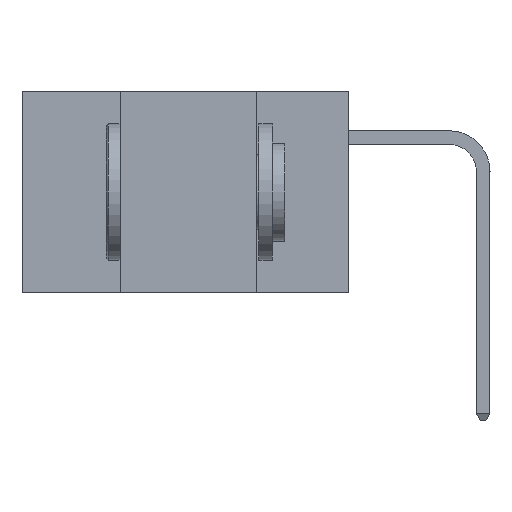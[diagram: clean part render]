
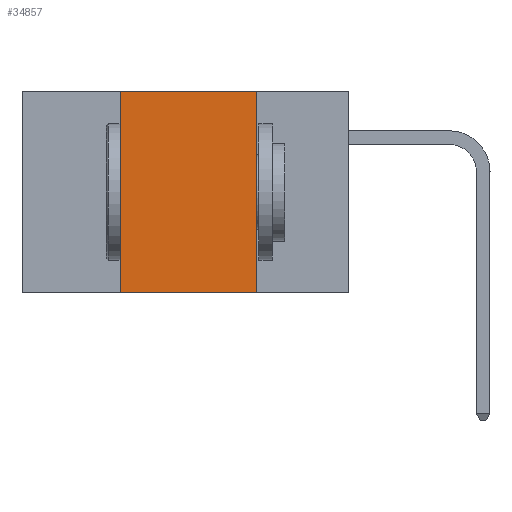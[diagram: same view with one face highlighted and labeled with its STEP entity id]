
A CAD part, left-side view. The second image highlights one B-rep face of the part: STEP entity #34857.
In plain terms, the highlighted planar face has unit normal (-1, 0, 0).
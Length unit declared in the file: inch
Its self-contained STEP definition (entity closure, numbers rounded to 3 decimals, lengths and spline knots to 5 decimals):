
#494 = LINE ( 'NONE', #39666, #38726 ) ;
#1566 = CARTESIAN_POINT ( 'NONE',  ( 0., 0.42, -0.37 ) ) ;
#3999 = VECTOR ( 'NONE', #14563, 39.37008 ) ;
#4906 = EDGE_CURVE ( 'NONE', #32123, #40632, #26420, .T. ) ;
#5770 = LINE ( 'NONE', #21380, #45044 ) ;
#10221 = AXIS2_PLACEMENT_3D ( 'NONE', #17290, #43224, #21131 ) ;
#13733 = PLANE ( 'NONE',  #10221 ) ;
#14563 = DIRECTION ( 'NONE',  ( 0., -1., 0. ) ) ;
#15925 = ORIENTED_EDGE ( 'NONE', *, *, #32417, .F. ) ;
#17290 = CARTESIAN_POINT ( 'NONE',  ( 0., 0.6, 0. ) ) ;
#19367 = EDGE_LOOP ( 'NONE', ( #20616, #15925, #19670, #27482 ) ) ;
#19670 = ORIENTED_EDGE ( 'NONE', *, *, #33658, .F. ) ;
#20616 = ORIENTED_EDGE ( 'NONE', *, *, #44656, .F. ) ;
#21131 = DIRECTION ( 'NONE',  ( 0., 0., -1. ) ) ;
#21380 = CARTESIAN_POINT ( 'NONE',  ( 0., 0.42, 0. ) ) ;
#22202 = CARTESIAN_POINT ( 'NONE',  ( 0., 0.42, 0. ) ) ;
#25004 = DIRECTION ( 'NONE',  ( 0., 0., -1. ) ) ;
#26420 = LINE ( 'NONE', #29782, #35036 ) ;
#27482 = ORIENTED_EDGE ( 'NONE', *, *, #4906, .T. ) ;
#28075 = CARTESIAN_POINT ( 'NONE',  ( 0., 0.17, -0.37 ) ) ;
#28185 = CARTESIAN_POINT ( 'NONE',  ( 0., 0.17, 0. ) ) ;
#29782 = CARTESIAN_POINT ( 'NONE',  ( 0., 0.6, -0.37 ) ) ;
#32123 = VERTEX_POINT ( 'NONE', #1566 ) ;
#32417 = EDGE_CURVE ( 'NONE', #36283, #41343, #42188, .T. ) ;
#33658 = EDGE_CURVE ( 'NONE', #32123, #36283, #5770, .T. ) ;
#34857 = ADVANCED_FACE ( 'NONE', ( #38551 ), #13733, .F. ) ;
#35036 = VECTOR ( 'NONE', #40934, 39.37008 ) ;
#36283 = VERTEX_POINT ( 'NONE', #22202 ) ;
#36633 = CARTESIAN_POINT ( 'NONE',  ( 0., 0.6, 0. ) ) ;
#38551 = FACE_OUTER_BOUND ( 'NONE', #19367, .T. ) ;
#38726 = VECTOR ( 'NONE', #25004, 39.37008 ) ;
#39666 = CARTESIAN_POINT ( 'NONE',  ( 0., 0.17, 0. ) ) ;
#40632 = VERTEX_POINT ( 'NONE', #28075 ) ;
#40934 = DIRECTION ( 'NONE',  ( 0., -1., 0. ) ) ;
#41343 = VERTEX_POINT ( 'NONE', #28185 ) ;
#42188 = LINE ( 'NONE', #36633, #3999 ) ;
#43224 = DIRECTION ( 'NONE',  ( 1., 0., 0. ) ) ;
#44656 = EDGE_CURVE ( 'NONE', #41343, #40632, #494, .T. ) ;
#45044 = VECTOR ( 'NONE', #47178, 39.37008 ) ;
#47178 = DIRECTION ( 'NONE',  ( 0., 0., 1. ) ) ;
